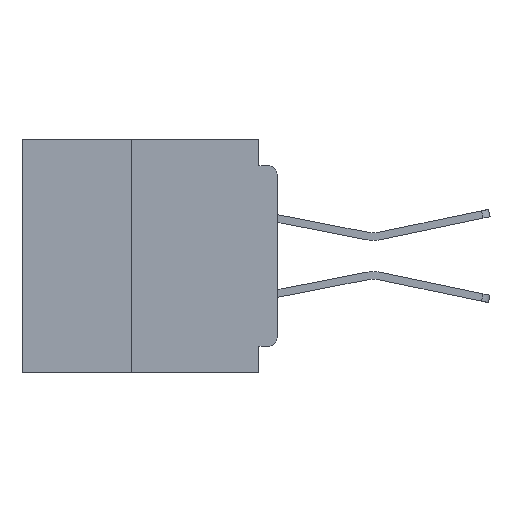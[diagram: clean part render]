
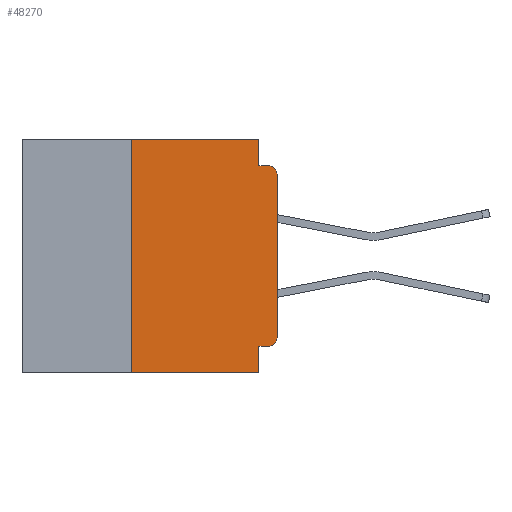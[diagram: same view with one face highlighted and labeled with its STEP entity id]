
A CAD part, left-side view. The second image highlights one B-rep face of the part: STEP entity #48270.
In plain terms, the highlighted planar face has unit normal (-1, 0, 0).
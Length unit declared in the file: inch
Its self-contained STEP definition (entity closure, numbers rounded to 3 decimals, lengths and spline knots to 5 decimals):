
#512 = VERTEX_POINT ( 'NONE', #41377 ) ;
#1114 = LINE ( 'NONE', #22117, #59101 ) ;
#1261 = EDGE_CURVE ( 'NONE', #11122, #2420, #19408, .T. ) ;
#2361 = EDGE_CURVE ( 'NONE', #3709, #512, #11762, .T. ) ;
#2420 = VERTEX_POINT ( 'NONE', #6793 ) ;
#3040 = CARTESIAN_POINT ( 'NONE',  ( 0., 0., -0.34 ) ) ;
#3279 = CARTESIAN_POINT ( 'NONE',  ( 0., 0.25, -0.4 ) ) ;
#3526 = EDGE_LOOP ( 'NONE', ( #20905, #17598, #20199, #15755, #6936, #21499, #41946, #5399, #45706, #56720 ) ) ;
#3677 = CARTESIAN_POINT ( 'NONE',  ( 0., 0.031, 0. ) ) ;
#3709 = VERTEX_POINT ( 'NONE', #53785 ) ;
#3863 = PLANE ( 'NONE',  #53923 ) ;
#4205 = VECTOR ( 'NONE', #11161, 39.37008 ) ;
#4731 = DIRECTION ( 'NONE',  ( 0., -1., 0. ) ) ;
#5399 = ORIENTED_EDGE ( 'NONE', *, *, #23693, .F. ) ;
#6379 = CARTESIAN_POINT ( 'NONE',  ( 0., 0.031, 0. ) ) ;
#6793 = CARTESIAN_POINT ( 'NONE',  ( 0., 0.015, -0.045 ) ) ;
#6936 = ORIENTED_EDGE ( 'NONE', *, *, #19683, .F. ) ;
#7428 = CARTESIAN_POINT ( 'NONE',  ( 0., 0.25, 0. ) ) ;
#7551 = VECTOR ( 'NONE', #53617, 39.37008 ) ;
#7809 = VERTEX_POINT ( 'NONE', #3040 ) ;
#7860 = LINE ( 'NONE', #59463, #56270 ) ;
#8022 = DIRECTION ( 'NONE',  ( 0., 0., 1. ) ) ;
#10547 = LINE ( 'NONE', #16625, #21568 ) ;
#10908 = DIRECTION ( 'NONE',  ( -1., 0., 0. ) ) ;
#11122 = VERTEX_POINT ( 'NONE', #48217 ) ;
#11161 = DIRECTION ( 'NONE',  ( 0., 0., -1. ) ) ;
#11762 = LINE ( 'NONE', #48434, #60122 ) ;
#11902 = LINE ( 'NONE', #3279, #35382 ) ;
#15529 = EDGE_CURVE ( 'NONE', #34415, #38939, #45006, .T. ) ;
#15755 = ORIENTED_EDGE ( 'NONE', *, *, #23511, .F. ) ;
#16258 = AXIS2_PLACEMENT_3D ( 'NONE', #26571, #59250, #31260 ) ;
#16347 = EDGE_CURVE ( 'NONE', #34415, #22109, #11902, .T. ) ;
#16625 = CARTESIAN_POINT ( 'NONE',  ( 0., 0., 0. ) ) ;
#17598 = ORIENTED_EDGE ( 'NONE', *, *, #18790, .T. ) ;
#18790 = EDGE_CURVE ( 'NONE', #22484, #2420, #35801, .T. ) ;
#19408 = LINE ( 'NONE', #51463, #41405 ) ;
#19683 = EDGE_CURVE ( 'NONE', #22109, #43854, #1114, .T. ) ;
#20158 = AXIS2_PLACEMENT_3D ( 'NONE', #38994, #10908, #43697 ) ;
#20199 = ORIENTED_EDGE ( 'NONE', *, *, #1261, .F. ) ;
#20581 = DIRECTION ( 'NONE',  ( 0., 1., 0. ) ) ;
#20905 = ORIENTED_EDGE ( 'NONE', *, *, #35646, .T. ) ;
#21499 = ORIENTED_EDGE ( 'NONE', *, *, #16347, .F. ) ;
#21568 = VECTOR ( 'NONE', #30821, 39.37008 ) ;
#22109 = VERTEX_POINT ( 'NONE', #7428 ) ;
#22117 = CARTESIAN_POINT ( 'NONE',  ( 0., 0.437, 0. ) ) ;
#22484 = VERTEX_POINT ( 'NONE', #47804 ) ;
#22846 = CARTESIAN_POINT ( 'NONE',  ( 0., 0.437, 0. ) ) ;
#23467 = FACE_OUTER_BOUND ( 'NONE', #3526, .T. ) ;
#23511 = EDGE_CURVE ( 'NONE', #43854, #11122, #41691, .T. ) ;
#23693 = EDGE_CURVE ( 'NONE', #512, #38939, #7860, .T. ) ;
#25646 = CARTESIAN_POINT ( 'NONE',  ( 0., 0.437, -0.4 ) ) ;
#26571 = CARTESIAN_POINT ( 'NONE',  ( 0., 0.015, -0.34 ) ) ;
#26878 = DIRECTION ( 'NONE',  ( 0., -1., 0. ) ) ;
#27604 = DIRECTION ( 'NONE',  ( 1., 0., 0. ) ) ;
#30821 = DIRECTION ( 'NONE',  ( 0., 0., 1. ) ) ;
#31260 = DIRECTION ( 'NONE',  ( 0., 0., -1. ) ) ;
#31474 = DIRECTION ( 'NONE',  ( 0., 0., -1. ) ) ;
#34415 = VERTEX_POINT ( 'NONE', #58314 ) ;
#35382 = VECTOR ( 'NONE', #8022, 39.37008 ) ;
#35646 = EDGE_CURVE ( 'NONE', #7809, #22484, #10547, .T. ) ;
#35801 = CIRCLE ( 'NONE', #20158, 0.015 ) ;
#38939 = VERTEX_POINT ( 'NONE', #53355 ) ;
#38994 = CARTESIAN_POINT ( 'NONE',  ( 0., 0.015, -0.06 ) ) ;
#41377 = CARTESIAN_POINT ( 'NONE',  ( 0., 0.031, -0.355 ) ) ;
#41405 = VECTOR ( 'NONE', #4731, 39.37008 ) ;
#41691 = LINE ( 'NONE', #6379, #4205 ) ;
#41946 = ORIENTED_EDGE ( 'NONE', *, *, #15529, .T. ) ;
#43697 = DIRECTION ( 'NONE',  ( 0., 0., -1. ) ) ;
#43854 = VERTEX_POINT ( 'NONE', #3677 ) ;
#45006 = LINE ( 'NONE', #25646, #7551 ) ;
#45706 = ORIENTED_EDGE ( 'NONE', *, *, #2361, .F. ) ;
#47804 = CARTESIAN_POINT ( 'NONE',  ( 0., 0., -0.06 ) ) ;
#48111 = EDGE_CURVE ( 'NONE', #3709, #7809, #55648, .T. ) ;
#48217 = CARTESIAN_POINT ( 'NONE',  ( 0., 0.031, -0.045 ) ) ;
#48270 = ADVANCED_FACE ( 'NONE', ( #23467 ), #3863, .F. ) ;
#48434 = CARTESIAN_POINT ( 'NONE',  ( 0., 0., -0.355 ) ) ;
#51463 = CARTESIAN_POINT ( 'NONE',  ( 0., 0., -0.045 ) ) ;
#53355 = CARTESIAN_POINT ( 'NONE',  ( 0., 0.031, -0.4 ) ) ;
#53617 = DIRECTION ( 'NONE',  ( 0., -1., 0. ) ) ;
#53785 = CARTESIAN_POINT ( 'NONE',  ( 0., 0.015, -0.355 ) ) ;
#53923 = AXIS2_PLACEMENT_3D ( 'NONE', #22846, #27604, #60249 ) ;
#55648 = CIRCLE ( 'NONE', #16258, 0.015 ) ;
#56270 = VECTOR ( 'NONE', #31474, 39.37008 ) ;
#56720 = ORIENTED_EDGE ( 'NONE', *, *, #48111, .T. ) ;
#58314 = CARTESIAN_POINT ( 'NONE',  ( 0., 0.25, -0.4 ) ) ;
#59101 = VECTOR ( 'NONE', #26878, 39.37008 ) ;
#59250 = DIRECTION ( 'NONE',  ( -1., 0., 0. ) ) ;
#59463 = CARTESIAN_POINT ( 'NONE',  ( 0., 0.031, -0.4 ) ) ;
#60122 = VECTOR ( 'NONE', #20581, 39.37008 ) ;
#60249 = DIRECTION ( 'NONE',  ( 0., 0., -1. ) ) ;
